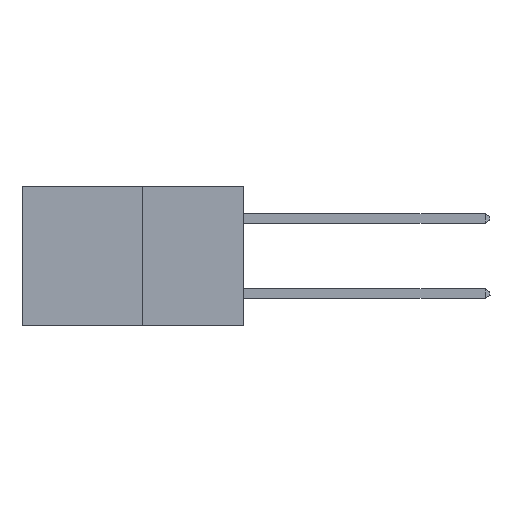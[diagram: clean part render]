
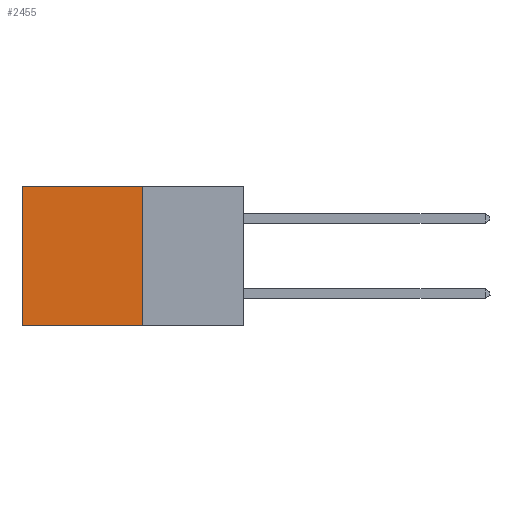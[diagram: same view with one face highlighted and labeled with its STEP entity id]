
A CAD part, left-side view. The second image highlights one B-rep face of the part: STEP entity #2455.
In plain terms, the highlighted planar face has unit normal (-1, 0, 0).
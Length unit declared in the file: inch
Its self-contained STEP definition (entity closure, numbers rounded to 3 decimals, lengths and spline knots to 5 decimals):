
#150 = LINE ( 'NONE', #569, #3524 ) ;
#349 = VECTOR ( 'NONE', #3722, 39.37008 ) ;
#569 = CARTESIAN_POINT ( 'NONE',  ( 0.277, 0.27, -0.37 ) ) ;
#727 = CARTESIAN_POINT ( 'NONE',  ( 0.277, 0.27, -0.37 ) ) ;
#743 = VERTEX_POINT ( 'NONE', #6011 ) ;
#918 = AXIS2_PLACEMENT_3D ( 'NONE', #727, #1516, #5493 ) ;
#955 = VECTOR ( 'NONE', #6412, 39.37008 ) ;
#1027 = DIRECTION ( 'NONE',  ( 0., 0., -1. ) ) ;
#1516 = DIRECTION ( 'NONE',  ( 1., 0., 0. ) ) ;
#1543 = CARTESIAN_POINT ( 'NONE',  ( 0.277, 0.27, 0. ) ) ;
#2455 = ADVANCED_FACE ( 'NONE', ( #7933 ), #7154, .F. ) ;
#2523 = ORIENTED_EDGE ( 'NONE', *, *, #7439, .T. ) ;
#2598 = EDGE_LOOP ( 'NONE', ( #2523, #6211, #6213, #6287 ) ) ;
#3481 = CARTESIAN_POINT ( 'NONE',  ( 0.277, 0.27, -0.37 ) ) ;
#3524 = VECTOR ( 'NONE', #1027, 39.37008 ) ;
#3550 = DIRECTION ( 'NONE',  ( 0., 1., 0. ) ) ;
#3722 = DIRECTION ( 'NONE',  ( 0., 0., -1. ) ) ;
#3726 = CARTESIAN_POINT ( 'NONE',  ( 0.277, 0.59, -0.37 ) ) ;
#3823 = VECTOR ( 'NONE', #3550, 39.37008 ) ;
#5213 = EDGE_CURVE ( 'NONE', #5808, #5991, #7572, .T. ) ;
#5476 = LINE ( 'NONE', #3726, #349 ) ;
#5493 = DIRECTION ( 'NONE',  ( 0., 0., -1. ) ) ;
#5582 = LINE ( 'NONE', #3481, #3823 ) ;
#5586 = EDGE_CURVE ( 'NONE', #743, #6653, #5582, .T. ) ;
#5808 = VERTEX_POINT ( 'NONE', #1543 ) ;
#5905 = EDGE_CURVE ( 'NONE', #5808, #743, #150, .T. ) ;
#5906 = CARTESIAN_POINT ( 'NONE',  ( 0.277, 0.59, -0.37 ) ) ;
#5991 = VERTEX_POINT ( 'NONE', #7956 ) ;
#6011 = CARTESIAN_POINT ( 'NONE',  ( 0.277, 0.27, -0.37 ) ) ;
#6211 = ORIENTED_EDGE ( 'NONE', *, *, #5586, .F. ) ;
#6213 = ORIENTED_EDGE ( 'NONE', *, *, #5905, .F. ) ;
#6287 = ORIENTED_EDGE ( 'NONE', *, *, #5213, .T. ) ;
#6412 = DIRECTION ( 'NONE',  ( 0., 1., 0. ) ) ;
#6552 = CARTESIAN_POINT ( 'NONE',  ( 0.277, 0.27, 0. ) ) ;
#6653 = VERTEX_POINT ( 'NONE', #5906 ) ;
#7154 = PLANE ( 'NONE',  #918 ) ;
#7439 = EDGE_CURVE ( 'NONE', #5991, #6653, #5476, .T. ) ;
#7572 = LINE ( 'NONE', #6552, #955 ) ;
#7933 = FACE_OUTER_BOUND ( 'NONE', #2598, .T. ) ;
#7956 = CARTESIAN_POINT ( 'NONE',  ( 0.277, 0.59, 0. ) ) ;
